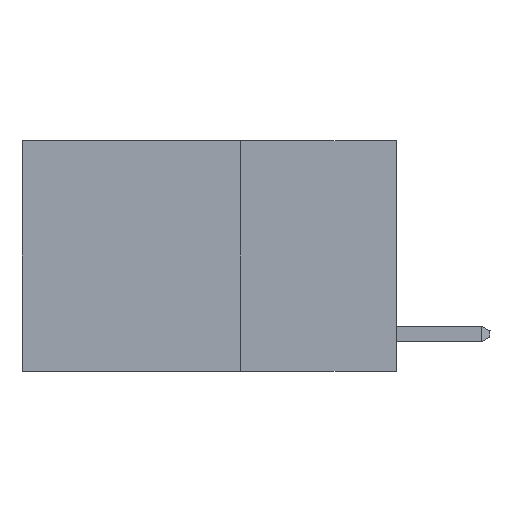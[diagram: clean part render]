
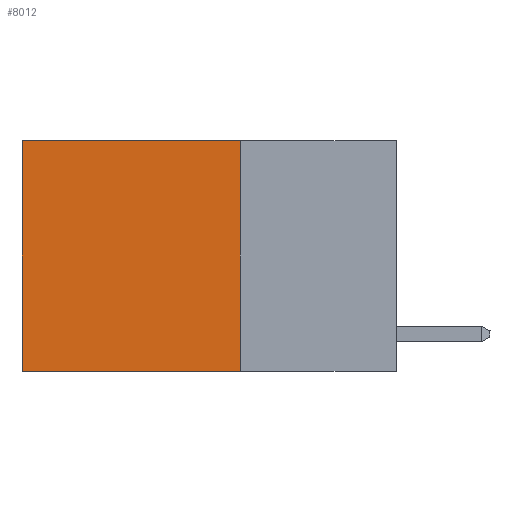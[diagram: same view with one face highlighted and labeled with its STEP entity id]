
A CAD part, left-side view. The second image highlights one B-rep face of the part: STEP entity #8012.
In plain terms, the highlighted planar face has unit normal (-1, 0, 0).
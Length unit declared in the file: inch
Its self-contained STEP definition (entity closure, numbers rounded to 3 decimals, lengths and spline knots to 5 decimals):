
#706 = EDGE_LOOP ( 'NONE', ( #3226, #8466, #5698, #15021 ) ) ;
#1344 = DIRECTION ( 'NONE',  ( 0., 0., -1. ) ) ;
#1587 = DIRECTION ( 'NONE',  ( 0., 1., 0. ) ) ;
#1960 = CARTESIAN_POINT ( 'NONE',  ( 0.2625, 0.25, -0.37 ) ) ;
#3003 = VECTOR ( 'NONE', #8484, 39.37008 ) ;
#3205 = LINE ( 'NONE', #7139, #3003 ) ;
#3226 = ORIENTED_EDGE ( 'NONE', *, *, #8273, .T. ) ;
#3661 = VECTOR ( 'NONE', #1344, 39.37008 ) ;
#4292 = VERTEX_POINT ( 'NONE', #14277 ) ;
#4406 = CARTESIAN_POINT ( 'NONE',  ( 0.2625, 0.25, 0. ) ) ;
#4742 = VERTEX_POINT ( 'NONE', #4406 ) ;
#5186 = EDGE_CURVE ( 'NONE', #4742, #4292, #5619, .T. ) ;
#5556 = AXIS2_PLACEMENT_3D ( 'NONE', #11711, #15707, #10458 ) ;
#5619 = LINE ( 'NONE', #13235, #12175 ) ;
#5698 = ORIENTED_EDGE ( 'NONE', *, *, #8443, .F. ) ;
#6295 = LINE ( 'NONE', #9291, #3661 ) ;
#7139 = CARTESIAN_POINT ( 'NONE',  ( 0.2625, 0.25, -0.37 ) ) ;
#7710 = VERTEX_POINT ( 'NONE', #8458 ) ;
#8012 = ADVANCED_FACE ( 'NONE', ( #9564 ), #11589, .F. ) ;
#8273 = EDGE_CURVE ( 'NONE', #4292, #7710, #14039, .T. ) ;
#8443 = EDGE_CURVE ( 'NONE', #4742, #13242, #6295, .T. ) ;
#8458 = CARTESIAN_POINT ( 'NONE',  ( 0.2625, 0.6, -0.37 ) ) ;
#8466 = ORIENTED_EDGE ( 'NONE', *, *, #11929, .F. ) ;
#8484 = DIRECTION ( 'NONE',  ( 0., 1., 0. ) ) ;
#9291 = CARTESIAN_POINT ( 'NONE',  ( 0.2625, 0.25, 0. ) ) ;
#9564 = FACE_OUTER_BOUND ( 'NONE', #706, .T. ) ;
#10458 = DIRECTION ( 'NONE',  ( 0., 0., -1. ) ) ;
#11589 = PLANE ( 'NONE',  #5556 ) ;
#11711 = CARTESIAN_POINT ( 'NONE',  ( 0.2625, 0.25, 0. ) ) ;
#11929 = EDGE_CURVE ( 'NONE', #13242, #7710, #3205, .T. ) ;
#12175 = VECTOR ( 'NONE', #1587, 39.37008 ) ;
#12816 = DIRECTION ( 'NONE',  ( 0., 0., -1. ) ) ;
#13235 = CARTESIAN_POINT ( 'NONE',  ( 0.2625, 0.25, 0. ) ) ;
#13242 = VERTEX_POINT ( 'NONE', #1960 ) ;
#13835 = VECTOR ( 'NONE', #12816, 39.37008 ) ;
#14039 = LINE ( 'NONE', #14209, #13835 ) ;
#14209 = CARTESIAN_POINT ( 'NONE',  ( 0.2625, 0.6, 0. ) ) ;
#14277 = CARTESIAN_POINT ( 'NONE',  ( 0.2625, 0.6, 0. ) ) ;
#15021 = ORIENTED_EDGE ( 'NONE', *, *, #5186, .T. ) ;
#15707 = DIRECTION ( 'NONE',  ( 1., 0., 0. ) ) ;
